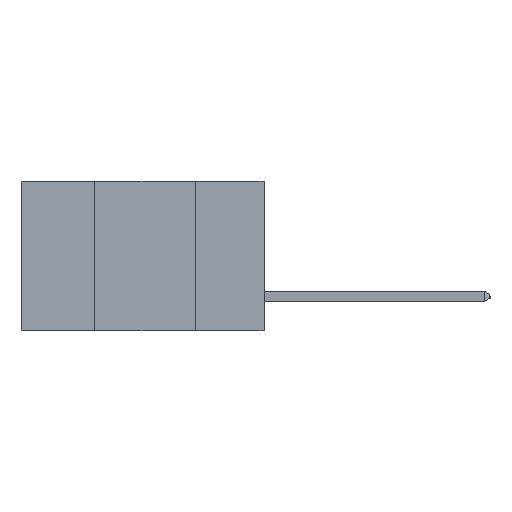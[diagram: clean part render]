
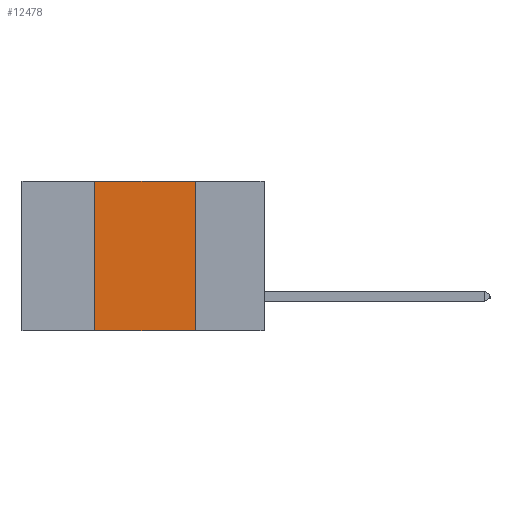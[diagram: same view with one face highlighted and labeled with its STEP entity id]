
A CAD part, left-side view. The second image highlights one B-rep face of the part: STEP entity #12478.
In plain terms, the highlighted planar face has unit normal (-1, 0, 0).
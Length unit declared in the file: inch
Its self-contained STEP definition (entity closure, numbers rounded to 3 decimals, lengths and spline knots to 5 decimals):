
#268 = CARTESIAN_POINT ( 'NONE',  ( 0., 0.17, 0. ) ) ;
#769 = DIRECTION ( 'NONE',  ( 1., 0., 0. ) ) ;
#799 = VECTOR ( 'NONE', #7817, 39.37008 ) ;
#1888 = AXIS2_PLACEMENT_3D ( 'NONE', #10466, #769, #9302 ) ;
#2218 = ORIENTED_EDGE ( 'NONE', *, *, #3946, .F. ) ;
#2263 = EDGE_CURVE ( 'NONE', #2302, #3814, #7023, .T. ) ;
#2302 = VERTEX_POINT ( 'NONE', #13345 ) ;
#3031 = ORIENTED_EDGE ( 'NONE', *, *, #2263, .F. ) ;
#3099 = VECTOR ( 'NONE', #14711, 39.37008 ) ;
#3814 = VERTEX_POINT ( 'NONE', #14668 ) ;
#3946 = EDGE_CURVE ( 'NONE', #12142, #4428, #10531, .T. ) ;
#4428 = VERTEX_POINT ( 'NONE', #15278 ) ;
#4678 = EDGE_CURVE ( 'NONE', #3814, #12142, #6385, .T. ) ;
#5303 = VECTOR ( 'NONE', #9031, 39.37008 ) ;
#5642 = EDGE_LOOP ( 'NONE', ( #2218, #11855, #3031, #9476 ) ) ;
#6168 = FACE_OUTER_BOUND ( 'NONE', #5642, .T. ) ;
#6385 = LINE ( 'NONE', #13961, #3099 ) ;
#6651 = CARTESIAN_POINT ( 'NONE',  ( 0., 0.6, -0.37 ) ) ;
#7023 = LINE ( 'NONE', #8949, #10202 ) ;
#7139 = DIRECTION ( 'NONE',  ( 0., 0., 1. ) ) ;
#7817 = DIRECTION ( 'NONE',  ( 0., 0., -1. ) ) ;
#8111 = PLANE ( 'NONE',  #1888 ) ;
#8520 = LINE ( 'NONE', #6651, #5303 ) ;
#8949 = CARTESIAN_POINT ( 'NONE',  ( 0., 0.42, 0. ) ) ;
#9031 = DIRECTION ( 'NONE',  ( 0., -1., 0. ) ) ;
#9302 = DIRECTION ( 'NONE',  ( 0., 0., -1. ) ) ;
#9476 = ORIENTED_EDGE ( 'NONE', *, *, #14224, .T. ) ;
#9602 = CARTESIAN_POINT ( 'NONE',  ( 0., 0.17, 0. ) ) ;
#10202 = VECTOR ( 'NONE', #7139, 39.37008 ) ;
#10466 = CARTESIAN_POINT ( 'NONE',  ( 0., 0.6, 0. ) ) ;
#10531 = LINE ( 'NONE', #268, #799 ) ;
#11855 = ORIENTED_EDGE ( 'NONE', *, *, #4678, .F. ) ;
#12142 = VERTEX_POINT ( 'NONE', #9602 ) ;
#12478 = ADVANCED_FACE ( 'NONE', ( #6168 ), #8111, .F. ) ;
#13345 = CARTESIAN_POINT ( 'NONE',  ( 0., 0.42, -0.37 ) ) ;
#13961 = CARTESIAN_POINT ( 'NONE',  ( 0., 0.6, 0. ) ) ;
#14224 = EDGE_CURVE ( 'NONE', #2302, #4428, #8520, .T. ) ;
#14668 = CARTESIAN_POINT ( 'NONE',  ( 0., 0.42, 0. ) ) ;
#14711 = DIRECTION ( 'NONE',  ( 0., -1., 0. ) ) ;
#15278 = CARTESIAN_POINT ( 'NONE',  ( 0., 0.17, -0.37 ) ) ;
